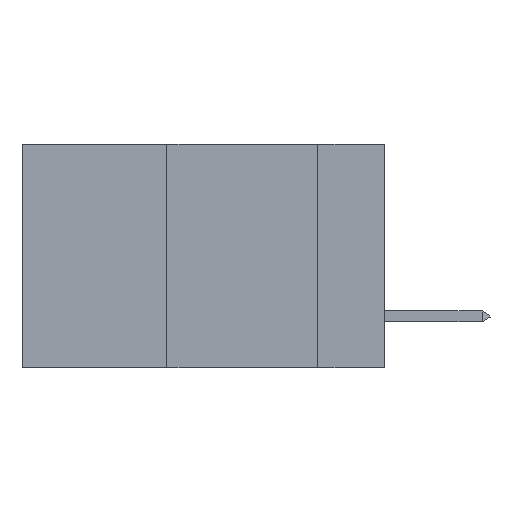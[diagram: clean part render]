
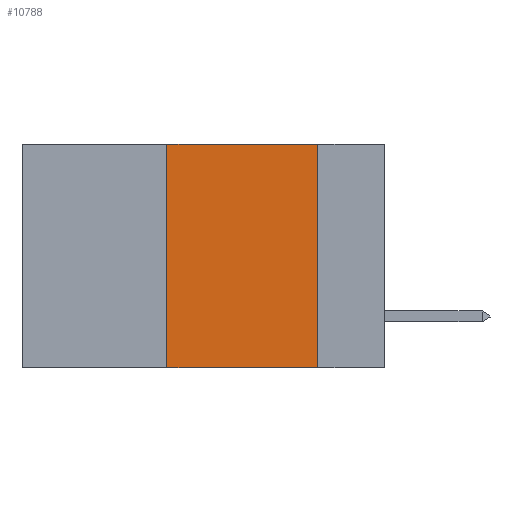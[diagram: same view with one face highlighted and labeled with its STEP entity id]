
A CAD part, left-side view. The second image highlights one B-rep face of the part: STEP entity #10788.
In plain terms, the highlighted planar face has unit normal (-1, 0, 0).
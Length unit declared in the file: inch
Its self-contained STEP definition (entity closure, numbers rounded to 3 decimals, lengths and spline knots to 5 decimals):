
#173 = CARTESIAN_POINT ( 'NONE',  ( 0., 0.36, -0.37 ) ) ;
#205 = DIRECTION ( 'NONE',  ( 0., -1., 0. ) ) ;
#251 = CARTESIAN_POINT ( 'NONE',  ( 0., 0.11, -0.37 ) ) ;
#684 = ORIENTED_EDGE ( 'NONE', *, *, #2791, .F. ) ;
#777 = DIRECTION ( 'NONE',  ( 0., -1., 0. ) ) ;
#1514 = VERTEX_POINT ( 'NONE', #251 ) ;
#1649 = DIRECTION ( 'NONE',  ( 0., 0., -1. ) ) ;
#2183 = EDGE_LOOP ( 'NONE', ( #684, #12906, #3224, #12238 ) ) ;
#2791 = EDGE_CURVE ( 'NONE', #11464, #1514, #8531, .T. ) ;
#3085 = CARTESIAN_POINT ( 'NONE',  ( 0., 0.11, 0. ) ) ;
#3194 = VECTOR ( 'NONE', #205, 39.37008 ) ;
#3224 = ORIENTED_EDGE ( 'NONE', *, *, #8173, .F. ) ;
#3807 = VECTOR ( 'NONE', #777, 39.37008 ) ;
#4121 = FACE_OUTER_BOUND ( 'NONE', #2183, .T. ) ;
#4817 = CARTESIAN_POINT ( 'NONE',  ( 0., 0.6, 0. ) ) ;
#5012 = VERTEX_POINT ( 'NONE', #173 ) ;
#5844 = VECTOR ( 'NONE', #1649, 39.37008 ) ;
#5852 = CARTESIAN_POINT ( 'NONE',  ( 0., 0.36, 0. ) ) ;
#6398 = LINE ( 'NONE', #6959, #3194 ) ;
#6959 = CARTESIAN_POINT ( 'NONE',  ( 0., 0.6, 0. ) ) ;
#7504 = AXIS2_PLACEMENT_3D ( 'NONE', #4817, #7874, #11958 ) ;
#7761 = CARTESIAN_POINT ( 'NONE',  ( 0., 0.6, -0.37 ) ) ;
#7874 = DIRECTION ( 'NONE',  ( 1., 0., 0. ) ) ;
#7954 = PLANE ( 'NONE',  #7504 ) ;
#8153 = VECTOR ( 'NONE', #12633, 39.37008 ) ;
#8173 = EDGE_CURVE ( 'NONE', #5012, #10310, #11214, .T. ) ;
#8531 = LINE ( 'NONE', #8934, #5844 ) ;
#8790 = EDGE_CURVE ( 'NONE', #10310, #11464, #6398, .T. ) ;
#8934 = CARTESIAN_POINT ( 'NONE',  ( 0., 0.11, 0. ) ) ;
#10310 = VERTEX_POINT ( 'NONE', #10536 ) ;
#10536 = CARTESIAN_POINT ( 'NONE',  ( 0., 0.36, 0. ) ) ;
#10788 = ADVANCED_FACE ( 'NONE', ( #4121 ), #7954, .F. ) ;
#11214 = LINE ( 'NONE', #5852, #8153 ) ;
#11464 = VERTEX_POINT ( 'NONE', #3085 ) ;
#11958 = DIRECTION ( 'NONE',  ( 0., 0., -1. ) ) ;
#12006 = LINE ( 'NONE', #7761, #3807 ) ;
#12238 = ORIENTED_EDGE ( 'NONE', *, *, #12504, .T. ) ;
#12504 = EDGE_CURVE ( 'NONE', #5012, #1514, #12006, .T. ) ;
#12633 = DIRECTION ( 'NONE',  ( 0., 0., 1. ) ) ;
#12906 = ORIENTED_EDGE ( 'NONE', *, *, #8790, .F. ) ;
